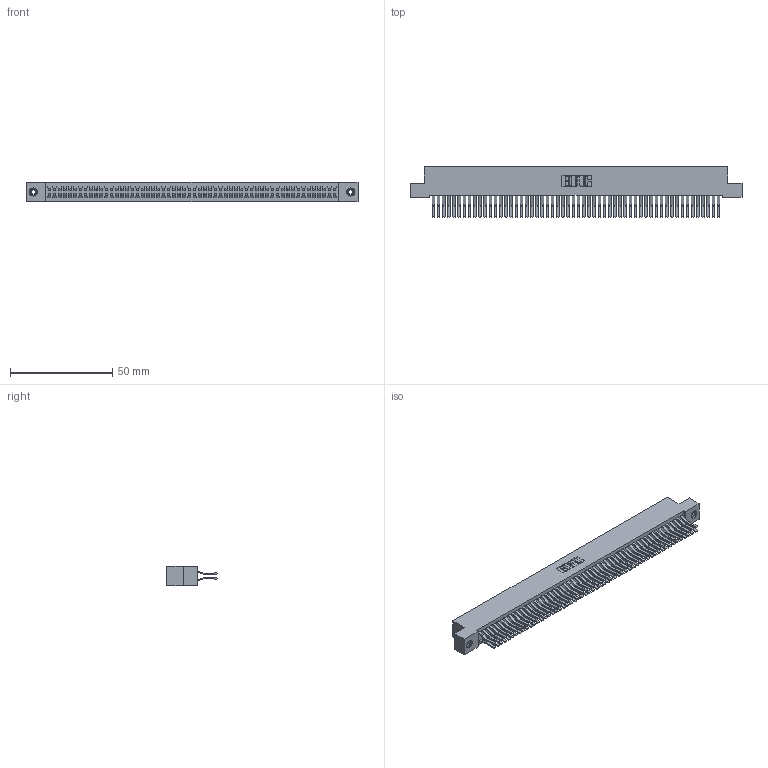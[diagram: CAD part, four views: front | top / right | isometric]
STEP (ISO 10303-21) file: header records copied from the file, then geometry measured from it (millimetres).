
FILE_DESCRIPTION (( 'STEP AP203' ), '1' );
FILE_NAME ('392-112-560-208.STEP', '2018-08-18T22:57:54', ( '' ), ( '' ), 'SwSTEP 2.0', 'SolidWorks 2016', '' );
FILE_SCHEMA (( 'CONFIG_CONTROL_DESIGN' ));
Length unit declared in the file: inch
Products named in the file (4): 392-112-560-208; 342 Part_TI; 345-292-001_560 Tail; 345-250-001_345-250-003-102
Assembly tree (115 placements, depth 2):
  392-112-560-208
    342 Part_TI
    345-292-001_560 Tail  x112
    345-250-001_345-250-003-102  x2
Bounding box: 162.56 x 24.78 x 9.4 mm (x, y, z)
Volume: 15401.9 mm3; surface area: 27188.9 mm2
Topology: 115 solids, 115 shells, 6218 faces, 18467 edges, 12154 vertices
Faces by surface type: plane 4130, cylinder 2072, cone 12, torus 4
Entity records: 35358 total; most frequent: CARTESIAN_POINT 5825, ORIENTED_EDGE 5754, DIRECTION 4987, EDGE_CURVE 2877, VECTOR 2725, LINE 2725, VERTEX_POINT 1912, AXIS2_PLACEMENT_3D 1131
